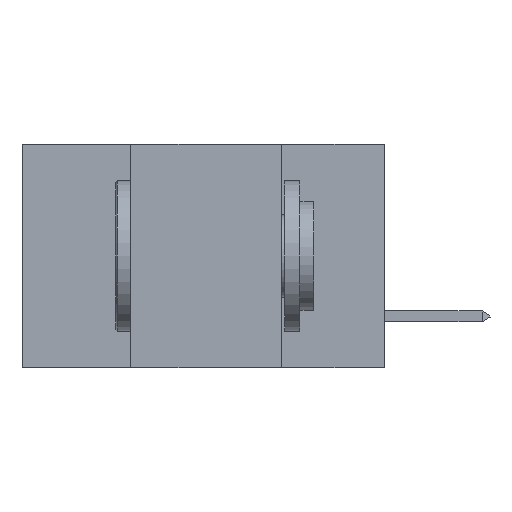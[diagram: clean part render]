
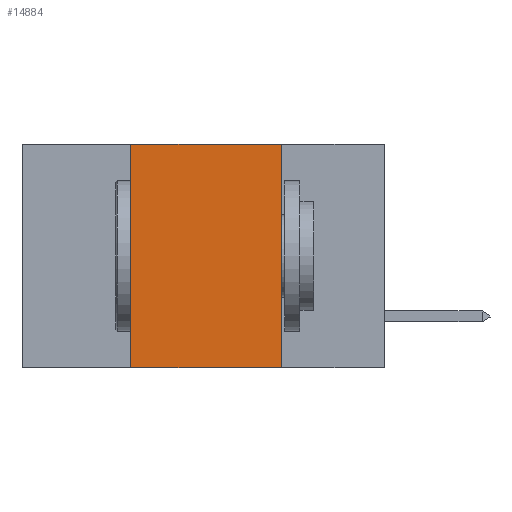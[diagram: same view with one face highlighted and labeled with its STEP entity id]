
A CAD part, left-side view. The second image highlights one B-rep face of the part: STEP entity #14884.
In plain terms, the highlighted planar face has unit normal (-1, 0, 0).
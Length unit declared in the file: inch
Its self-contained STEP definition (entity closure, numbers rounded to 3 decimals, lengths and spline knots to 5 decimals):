
#240 = CARTESIAN_POINT ( 'NONE',  ( 0., 0.42, 0. ) ) ;
#1126 = AXIS2_PLACEMENT_3D ( 'NONE', #35861, #35378, #27004 ) ;
#3320 = CARTESIAN_POINT ( 'NONE',  ( 0., 0.17, 0. ) ) ;
#3849 = CARTESIAN_POINT ( 'NONE',  ( 0., 0.42, -0.37 ) ) ;
#4306 = PLANE ( 'NONE',  #1126 ) ;
#4437 = CARTESIAN_POINT ( 'NONE',  ( 0., 0.6, -0.37 ) ) ;
#4746 = DIRECTION ( 'NONE',  ( 0., -1., 0. ) ) ;
#5668 = VERTEX_POINT ( 'NONE', #3849 ) ;
#5691 = FACE_OUTER_BOUND ( 'NONE', #7160, .T. ) ;
#7160 = EDGE_LOOP ( 'NONE', ( #28254, #15055, #8447, #11085 ) ) ;
#7258 = EDGE_CURVE ( 'NONE', #5668, #20806, #16731, .T. ) ;
#8442 = EDGE_CURVE ( 'NONE', #5668, #17589, #17800, .T. ) ;
#8447 = ORIENTED_EDGE ( 'NONE', *, *, #7258, .F. ) ;
#9321 = DIRECTION ( 'NONE',  ( 0., 0., -1. ) ) ;
#11006 = CARTESIAN_POINT ( 'NONE',  ( 0., 0.17, -0.37 ) ) ;
#11085 = ORIENTED_EDGE ( 'NONE', *, *, #8442, .T. ) ;
#12124 = VECTOR ( 'NONE', #9321, 39.37008 ) ;
#14884 = ADVANCED_FACE ( 'NONE', ( #5691 ), #4306, .F. ) ;
#15035 = CARTESIAN_POINT ( 'NONE',  ( 0., 0.17, 0. ) ) ;
#15055 = ORIENTED_EDGE ( 'NONE', *, *, #30819, .F. ) ;
#16148 = CARTESIAN_POINT ( 'NONE',  ( 0., 0.6, 0. ) ) ;
#16731 = LINE ( 'NONE', #240, #20253 ) ;
#17331 = EDGE_CURVE ( 'NONE', #19584, #17589, #30326, .T. ) ;
#17589 = VERTEX_POINT ( 'NONE', #11006 ) ;
#17800 = LINE ( 'NONE', #4437, #25821 ) ;
#19584 = VERTEX_POINT ( 'NONE', #3320 ) ;
#20253 = VECTOR ( 'NONE', #36672, 39.37008 ) ;
#20524 = CARTESIAN_POINT ( 'NONE',  ( 0., 0.42, 0. ) ) ;
#20806 = VERTEX_POINT ( 'NONE', #20524 ) ;
#24289 = DIRECTION ( 'NONE',  ( 0., -1., 0. ) ) ;
#25821 = VECTOR ( 'NONE', #24289, 39.37008 ) ;
#27004 = DIRECTION ( 'NONE',  ( 0., 0., -1. ) ) ;
#28254 = ORIENTED_EDGE ( 'NONE', *, *, #17331, .F. ) ;
#29668 = VECTOR ( 'NONE', #4746, 39.37008 ) ;
#30326 = LINE ( 'NONE', #15035, #12124 ) ;
#30819 = EDGE_CURVE ( 'NONE', #20806, #19584, #33264, .T. ) ;
#33264 = LINE ( 'NONE', #16148, #29668 ) ;
#35378 = DIRECTION ( 'NONE',  ( 1., 0., 0. ) ) ;
#35861 = CARTESIAN_POINT ( 'NONE',  ( 0., 0.6, 0. ) ) ;
#36672 = DIRECTION ( 'NONE',  ( 0., 0., 1. ) ) ;
